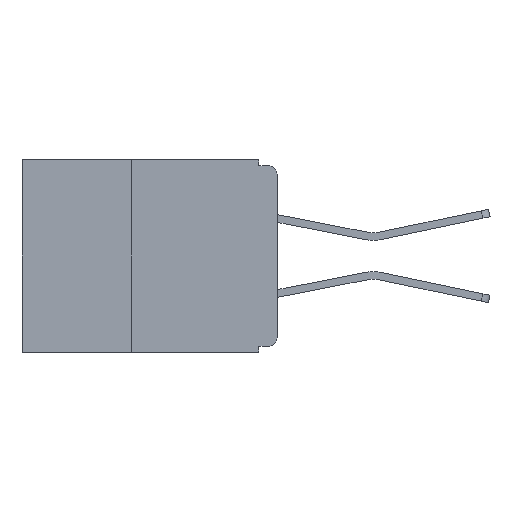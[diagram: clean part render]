
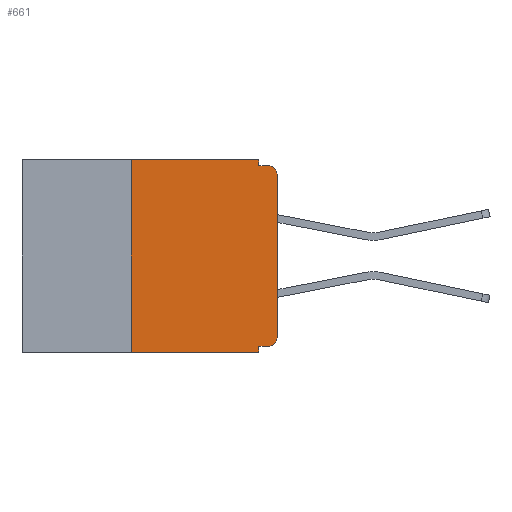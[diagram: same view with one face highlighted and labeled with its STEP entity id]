
A CAD part, left-side view. The second image highlights one B-rep face of the part: STEP entity #661.
In plain terms, the highlighted planar face has unit normal (-1, 0, 0).
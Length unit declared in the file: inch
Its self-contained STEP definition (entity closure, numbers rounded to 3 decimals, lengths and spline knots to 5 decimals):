
#96 = EDGE_CURVE ( 'NONE', #6663, #18389, #411, .T. ) ;
#411 = LINE ( 'NONE', #6141, #17359 ) ;
#661 = ADVANCED_FACE ( 'NONE', ( #6560 ), #13675, .F. ) ;
#905 = DIRECTION ( 'NONE',  ( 0., 0., 1. ) ) ;
#1220 = DIRECTION ( 'NONE',  ( 0., 0., -1. ) ) ;
#1862 = DIRECTION ( 'NONE',  ( -1., 0., 0. ) ) ;
#1892 = CARTESIAN_POINT ( 'NONE',  ( 0., 0.015, -0.025 ) ) ;
#2126 = VECTOR ( 'NONE', #12284, 39.37008 ) ;
#2371 = CIRCLE ( 'NONE', #19049, 0.015 ) ;
#2818 = CARTESIAN_POINT ( 'NONE',  ( 0., 0., -0.025 ) ) ;
#2879 = EDGE_CURVE ( 'NONE', #20149, #10648, #2371, .T. ) ;
#2986 = ORIENTED_EDGE ( 'NONE', *, *, #2879, .T. ) ;
#3186 = DIRECTION ( 'NONE',  ( 0., 0., -1. ) ) ;
#3211 = EDGE_CURVE ( 'NONE', #14319, #6663, #17497, .T. ) ;
#3248 = ORIENTED_EDGE ( 'NONE', *, *, #3211, .F. ) ;
#3474 = DIRECTION ( 'NONE',  ( 0., 0., -1. ) ) ;
#3758 = ORIENTED_EDGE ( 'NONE', *, *, #11891, .T. ) ;
#3811 = ORIENTED_EDGE ( 'NONE', *, *, #19538, .F. ) ;
#3835 = DIRECTION ( 'NONE',  ( 0., 1., 0. ) ) ;
#4123 = CARTESIAN_POINT ( 'NONE',  ( 0., 0.437, -0.33 ) ) ;
#4130 = LINE ( 'NONE', #13004, #16695 ) ;
#4133 = AXIS2_PLACEMENT_3D ( 'NONE', #20440, #12499, #20722 ) ;
#4466 = LINE ( 'NONE', #15289, #16003 ) ;
#4502 = CARTESIAN_POINT ( 'NONE',  ( 0., 0.015, -0.01 ) ) ;
#4620 = DIRECTION ( 'NONE',  ( 1., 0., 0. ) ) ;
#4729 = EDGE_CURVE ( 'NONE', #13878, #7334, #10260, .T. ) ;
#5298 = ORIENTED_EDGE ( 'NONE', *, *, #9412, .F. ) ;
#6141 = CARTESIAN_POINT ( 'NONE',  ( 0., 0.437, 0. ) ) ;
#6462 = CARTESIAN_POINT ( 'NONE',  ( 0., 0.031, -0.01 ) ) ;
#6560 = FACE_OUTER_BOUND ( 'NONE', #16662, .T. ) ;
#6663 = VERTEX_POINT ( 'NONE', #9882 ) ;
#6756 = VERTEX_POINT ( 'NONE', #6462 ) ;
#7334 = VERTEX_POINT ( 'NONE', #16849 ) ;
#7518 = LINE ( 'NONE', #4123, #2126 ) ;
#7601 = DIRECTION ( 'NONE',  ( 0., -1., 0. ) ) ;
#7839 = CARTESIAN_POINT ( 'NONE',  ( 0., 0.031, -0.33 ) ) ;
#8887 = CARTESIAN_POINT ( 'NONE',  ( 0., 0.25, -0.33 ) ) ;
#9032 = VERTEX_POINT ( 'NONE', #13041 ) ;
#9246 = EDGE_CURVE ( 'NONE', #14319, #9032, #7518, .T. ) ;
#9412 = EDGE_CURVE ( 'NONE', #19609, #9032, #20321, .T. ) ;
#9732 = VECTOR ( 'NONE', #11080, 39.37008 ) ;
#9882 = CARTESIAN_POINT ( 'NONE',  ( 0., 0.25, 0. ) ) ;
#10255 = LINE ( 'NONE', #19267, #9732 ) ;
#10260 = CIRCLE ( 'NONE', #4133, 0.015 ) ;
#10648 = VERTEX_POINT ( 'NONE', #4502 ) ;
#10658 = ORIENTED_EDGE ( 'NONE', *, *, #96, .F. ) ;
#10895 = ORIENTED_EDGE ( 'NONE', *, *, #11714, .F. ) ;
#11080 = DIRECTION ( 'NONE',  ( 0., 0., -1. ) ) ;
#11606 = VECTOR ( 'NONE', #1220, 39.37008 ) ;
#11714 = EDGE_CURVE ( 'NONE', #6756, #10648, #12071, .T. ) ;
#11891 = EDGE_CURVE ( 'NONE', #7334, #20149, #4130, .T. ) ;
#12071 = LINE ( 'NONE', #19054, #15928 ) ;
#12284 = DIRECTION ( 'NONE',  ( 0., -1., 0. ) ) ;
#12499 = DIRECTION ( 'NONE',  ( -1., 0., 0. ) ) ;
#13004 = CARTESIAN_POINT ( 'NONE',  ( 0., 0., 0. ) ) ;
#13041 = CARTESIAN_POINT ( 'NONE',  ( 0., 0.031, -0.33 ) ) ;
#13177 = CARTESIAN_POINT ( 'NONE',  ( 0., 0.031, 0. ) ) ;
#13675 = PLANE ( 'NONE',  #20512 ) ;
#13795 = CARTESIAN_POINT ( 'NONE',  ( 0., 0.437, 0. ) ) ;
#13878 = VERTEX_POINT ( 'NONE', #21056 ) ;
#13992 = ORIENTED_EDGE ( 'NONE', *, *, #4729, .T. ) ;
#14319 = VERTEX_POINT ( 'NONE', #15921 ) ;
#15041 = DIRECTION ( 'NONE',  ( 0., -1., 0. ) ) ;
#15289 = CARTESIAN_POINT ( 'NONE',  ( 0., 0., -0.32 ) ) ;
#15921 = CARTESIAN_POINT ( 'NONE',  ( 0., 0.25, -0.33 ) ) ;
#15928 = VECTOR ( 'NONE', #7601, 39.37008 ) ;
#16003 = VECTOR ( 'NONE', #3835, 39.37008 ) ;
#16206 = CARTESIAN_POINT ( 'NONE',  ( 0., 0.031, -0.32 ) ) ;
#16580 = EDGE_CURVE ( 'NONE', #13878, #19609, #4466, .T. ) ;
#16662 = EDGE_LOOP ( 'NONE', ( #3758, #2986, #10895, #3811, #10658, #3248, #20662, #5298, #19122, #13992 ) ) ;
#16695 = VECTOR ( 'NONE', #21107, 39.37008 ) ;
#16849 = CARTESIAN_POINT ( 'NONE',  ( 0., 0., -0.305 ) ) ;
#16991 = VECTOR ( 'NONE', #905, 39.37008 ) ;
#17359 = VECTOR ( 'NONE', #15041, 39.37008 ) ;
#17497 = LINE ( 'NONE', #8887, #16991 ) ;
#18389 = VERTEX_POINT ( 'NONE', #13177 ) ;
#19049 = AXIS2_PLACEMENT_3D ( 'NONE', #1892, #1862, #3474 ) ;
#19054 = CARTESIAN_POINT ( 'NONE',  ( 0., 0., -0.01 ) ) ;
#19122 = ORIENTED_EDGE ( 'NONE', *, *, #16580, .F. ) ;
#19267 = CARTESIAN_POINT ( 'NONE',  ( 0., 0.031, 0. ) ) ;
#19538 = EDGE_CURVE ( 'NONE', #18389, #6756, #10255, .T. ) ;
#19609 = VERTEX_POINT ( 'NONE', #16206 ) ;
#20149 = VERTEX_POINT ( 'NONE', #2818 ) ;
#20321 = LINE ( 'NONE', #7839, #11606 ) ;
#20440 = CARTESIAN_POINT ( 'NONE',  ( 0., 0.015, -0.305 ) ) ;
#20512 = AXIS2_PLACEMENT_3D ( 'NONE', #13795, #4620, #3186 ) ;
#20662 = ORIENTED_EDGE ( 'NONE', *, *, #9246, .T. ) ;
#20722 = DIRECTION ( 'NONE',  ( 0., 0., -1. ) ) ;
#21056 = CARTESIAN_POINT ( 'NONE',  ( 0., 0.015, -0.32 ) ) ;
#21107 = DIRECTION ( 'NONE',  ( 0., 0., 1. ) ) ;
